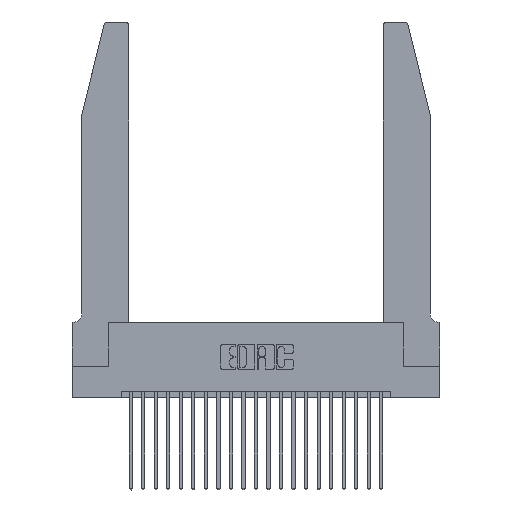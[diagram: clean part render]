
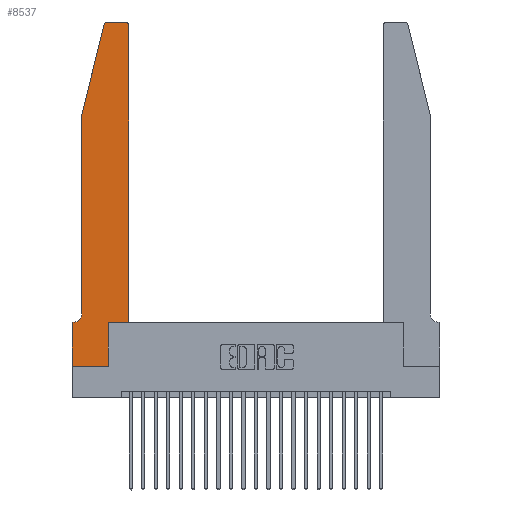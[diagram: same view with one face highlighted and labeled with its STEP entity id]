
A CAD part, top view. The second image highlights one B-rep face of the part: STEP entity #8537.
In plain terms, the highlighted planar face has unit normal (0, 0, 1).
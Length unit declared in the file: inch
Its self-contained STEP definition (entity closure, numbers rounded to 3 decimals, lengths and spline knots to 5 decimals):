
#343 = ORIENTED_EDGE ( 'NONE', *, *, #5346, .T. ) ;
#386 = EDGE_CURVE ( 'NONE', #7853, #14441, #5039, .T. ) ;
#389 = ORIENTED_EDGE ( 'NONE', *, *, #724, .T. ) ;
#724 = EDGE_CURVE ( 'NONE', #10968, #21668, #21007, .T. ) ;
#1003 = DIRECTION ( 'NONE',  ( -0.239, -0.971, 0. ) ) ;
#1478 = CARTESIAN_POINT ( 'NONE',  ( 0.0055, 0.35, 0.37 ) ) ;
#1730 = VECTOR ( 'NONE', #8742, 39.37008 ) ;
#1929 = CARTESIAN_POINT ( 'NONE',  ( 0.0755, 2., 0.37 ) ) ;
#2091 = DIRECTION ( 'NONE',  ( 1., 0., 0. ) ) ;
#2176 = CIRCLE ( 'NONE', #15638, 0.07 ) ;
#2273 = LINE ( 'NONE', #14148, #11302 ) ;
#2563 = EDGE_CURVE ( 'NONE', #12100, #7853, #19461, .T. ) ;
#3540 = DIRECTION ( 'NONE',  ( 1., 0., 0. ) ) ;
#3627 = LINE ( 'NONE', #9372, #23178 ) ;
#3744 = EDGE_CURVE ( 'NONE', #21668, #8141, #2273, .T. ) ;
#4007 = DIRECTION ( 'NONE',  ( 1., 0., 0. ) ) ;
#4068 = VERTEX_POINT ( 'NONE', #18173 ) ;
#4289 = CARTESIAN_POINT ( 'NONE',  ( 0.4505, 2.72, 0.37 ) ) ;
#4291 = DIRECTION ( 'NONE',  ( 0., 0., 1. ) ) ;
#4533 = CARTESIAN_POINT ( 'NONE',  ( 0.4205, 2.75, 0.37 ) ) ;
#4723 = VECTOR ( 'NONE', #1003, 39.37008 ) ;
#5039 = LINE ( 'NONE', #5408, #21942 ) ;
#5346 = EDGE_CURVE ( 'NONE', #8141, #5809, #2176, .T. ) ;
#5408 = CARTESIAN_POINT ( 'NONE',  ( 0.4505, 0.35, 0.37 ) ) ;
#5435 = CARTESIAN_POINT ( 'NONE',  ( 0.4505, 0.35, 0.37 ) ) ;
#5485 = EDGE_CURVE ( 'NONE', #4068, #10053, #19950, .T. ) ;
#5547 = VERTEX_POINT ( 'NONE', #4533 ) ;
#5669 = CARTESIAN_POINT ( 'NONE',  ( 0.2865, 0., 0.37 ) ) ;
#5801 = CIRCLE ( 'NONE', #22684, 0.03 ) ;
#5809 = VERTEX_POINT ( 'NONE', #1478 ) ;
#6621 = VERTEX_POINT ( 'NONE', #17341 ) ;
#6711 = CARTESIAN_POINT ( 'NONE',  ( 0.0755, 0.42, 0.37 ) ) ;
#6848 = VECTOR ( 'NONE', #18467, 39.37008 ) ;
#7501 = CARTESIAN_POINT ( 'NONE',  ( 0., 0.35, 0.37 ) ) ;
#7568 = PLANE ( 'NONE',  #18207 ) ;
#7853 = VERTEX_POINT ( 'NONE', #21515 ) ;
#8079 = EDGE_CURVE ( 'NONE', #5547, #6621, #10170, .T. ) ;
#8122 = CARTESIAN_POINT ( 'NONE',  ( 0.2865, 0.35, 0.37 ) ) ;
#8141 = VERTEX_POINT ( 'NONE', #6711 ) ;
#8286 = VECTOR ( 'NONE', #16804, 39.37008 ) ;
#8537 = ADVANCED_FACE ( 'NONE', ( #20017 ), #7568, .T. ) ;
#8742 = DIRECTION ( 'NONE',  ( -1., 0., 0. ) ) ;
#8786 = CARTESIAN_POINT ( 'NONE',  ( 0.0755, 0.35, 0.37 ) ) ;
#9141 = DIRECTION ( 'NONE',  ( 0., 0., 1. ) ) ;
#9211 = CIRCLE ( 'NONE', #14216, 0.03 ) ;
#9306 = ORIENTED_EDGE ( 'NONE', *, *, #2563, .T. ) ;
#9372 = CARTESIAN_POINT ( 'NONE',  ( 0., 0., 0.37 ) ) ;
#10053 = VERTEX_POINT ( 'NONE', #21650 ) ;
#10170 = LINE ( 'NONE', #19535, #1730 ) ;
#10679 = VERTEX_POINT ( 'NONE', #4289 ) ;
#10719 = DIRECTION ( 'NONE',  ( -1., 0., 0. ) ) ;
#10968 = VERTEX_POINT ( 'NONE', #15538 ) ;
#11052 = EDGE_CURVE ( 'NONE', #10053, #12100, #3627, .T. ) ;
#11302 = VECTOR ( 'NONE', #16076, 39.37008 ) ;
#11359 = ORIENTED_EDGE ( 'NONE', *, *, #5485, .T. ) ;
#11749 = ORIENTED_EDGE ( 'NONE', *, *, #17979, .T. ) ;
#11975 = EDGE_CURVE ( 'NONE', #5809, #4068, #23679, .T. ) ;
#12100 = VERTEX_POINT ( 'NONE', #5669 ) ;
#12582 = ORIENTED_EDGE ( 'NONE', *, *, #11052, .T. ) ;
#12632 = DIRECTION ( 'NONE',  ( 0., 0., -1. ) ) ;
#13716 = ORIENTED_EDGE ( 'NONE', *, *, #386, .T. ) ;
#14148 = CARTESIAN_POINT ( 'NONE',  ( 0.0755, 2., 0.37 ) ) ;
#14216 = AXIS2_PLACEMENT_3D ( 'NONE', #14719, #9141, #3540 ) ;
#14375 = EDGE_CURVE ( 'NONE', #10679, #5547, #5801, .T. ) ;
#14441 = VERTEX_POINT ( 'NONE', #23376 ) ;
#14719 = CARTESIAN_POINT ( 'NONE',  ( 0.284, 2.72, 0.37 ) ) ;
#14870 = VECTOR ( 'NONE', #19299, 39.37008 ) ;
#15167 = ORIENTED_EDGE ( 'NONE', *, *, #8079, .T. ) ;
#15538 = CARTESIAN_POINT ( 'NONE',  ( 0.25487, 2.72718, 0.37 ) ) ;
#15638 = AXIS2_PLACEMENT_3D ( 'NONE', #21688, #12632, #10719 ) ;
#15750 = ORIENTED_EDGE ( 'NONE', *, *, #3744, .T. ) ;
#16076 = DIRECTION ( 'NONE',  ( 0., -1., 0. ) ) ;
#16109 = CARTESIAN_POINT ( 'NONE',  ( 0.0755, 2., 0.37 ) ) ;
#16804 = DIRECTION ( 'NONE',  ( 0., -1., 0. ) ) ;
#17279 = CARTESIAN_POINT ( 'NONE',  ( 0., 0., 0.37 ) ) ;
#17341 = CARTESIAN_POINT ( 'NONE',  ( 0.284, 2.75, 0.37 ) ) ;
#17979 = EDGE_CURVE ( 'NONE', #14441, #10679, #21384, .T. ) ;
#18173 = CARTESIAN_POINT ( 'NONE',  ( 0., 0.35, 0.37 ) ) ;
#18207 = AXIS2_PLACEMENT_3D ( 'NONE', #7501, #22188, #2091 ) ;
#18467 = DIRECTION ( 'NONE',  ( 0., 1., 0. ) ) ;
#19255 = DIRECTION ( 'NONE',  ( 1., 0., 0. ) ) ;
#19299 = DIRECTION ( 'NONE',  ( 0., 1., 0. ) ) ;
#19461 = LINE ( 'NONE', #8122, #14870 ) ;
#19535 = CARTESIAN_POINT ( 'NONE',  ( 0.2605, 2.75, 0.37 ) ) ;
#19950 = LINE ( 'NONE', #17279, #8286 ) ;
#20017 = FACE_OUTER_BOUND ( 'NONE', #22604, .T. ) ;
#21007 = LINE ( 'NONE', #16109, #4723 ) ;
#21384 = LINE ( 'NONE', #5435, #6848 ) ;
#21515 = CARTESIAN_POINT ( 'NONE',  ( 0.2865, 0.35, 0.37 ) ) ;
#21611 = EDGE_CURVE ( 'NONE', #6621, #10968, #9211, .T. ) ;
#21650 = CARTESIAN_POINT ( 'NONE',  ( 0., 0., 0.37 ) ) ;
#21668 = VERTEX_POINT ( 'NONE', #1929 ) ;
#21688 = CARTESIAN_POINT ( 'NONE',  ( 0.0055, 0.42, 0.37 ) ) ;
#21825 = DIRECTION ( 'NONE',  ( -1., 0., 0. ) ) ;
#21875 = ORIENTED_EDGE ( 'NONE', *, *, #11975, .T. ) ;
#21939 = VECTOR ( 'NONE', #21825, 39.37008 ) ;
#21942 = VECTOR ( 'NONE', #4007, 39.37008 ) ;
#22188 = DIRECTION ( 'NONE',  ( 0., 0., 1. ) ) ;
#22221 = ORIENTED_EDGE ( 'NONE', *, *, #21611, .T. ) ;
#22349 = ORIENTED_EDGE ( 'NONE', *, *, #14375, .T. ) ;
#22417 = DIRECTION ( 'NONE',  ( 1., 0., 0. ) ) ;
#22604 = EDGE_LOOP ( 'NONE', ( #15167, #22221, #389, #15750, #343, #21875, #11359, #12582, #9306, #13716, #11749, #22349 ) ) ;
#22684 = AXIS2_PLACEMENT_3D ( 'NONE', #23140, #4291, #19255 ) ;
#23140 = CARTESIAN_POINT ( 'NONE',  ( 0.4205, 2.72, 0.37 ) ) ;
#23178 = VECTOR ( 'NONE', #22417, 39.37008 ) ;
#23376 = CARTESIAN_POINT ( 'NONE',  ( 0.4505, 0.35, 0.37 ) ) ;
#23679 = LINE ( 'NONE', #8786, #21939 ) ;
